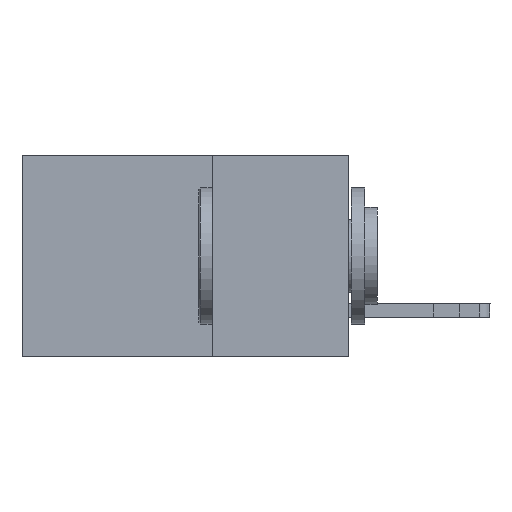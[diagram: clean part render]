
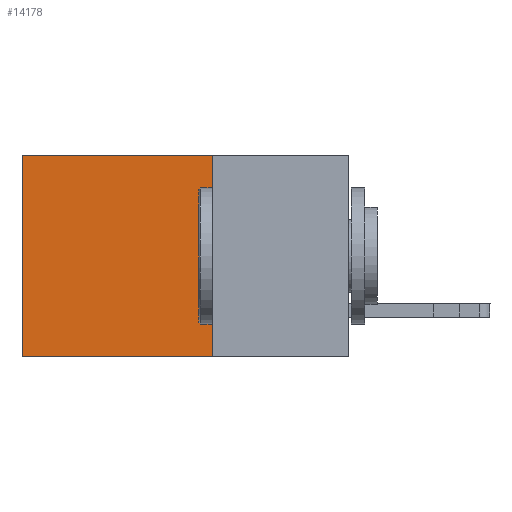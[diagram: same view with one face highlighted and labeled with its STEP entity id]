
A CAD part, left-side view. The second image highlights one B-rep face of the part: STEP entity #14178.
In plain terms, the highlighted planar face has unit normal (-1, 0, 0).
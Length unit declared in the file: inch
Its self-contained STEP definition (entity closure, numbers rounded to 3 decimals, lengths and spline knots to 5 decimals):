
#220 = VERTEX_POINT ( 'NONE', #11306 ) ;
#519 = EDGE_CURVE ( 'NONE', #220, #4418, #6284, .T. ) ;
#1216 = VECTOR ( 'NONE', #6121, 39.37008 ) ;
#1465 = CARTESIAN_POINT ( 'NONE',  ( 0.2615, 0.6, -0.37 ) ) ;
#1903 = DIRECTION ( 'NONE',  ( 1., 0., 0. ) ) ;
#2370 = VERTEX_POINT ( 'NONE', #6396 ) ;
#3082 = DIRECTION ( 'NONE',  ( 0., 1., 0. ) ) ;
#3368 = CARTESIAN_POINT ( 'NONE',  ( 0.2615, 0.25, -0.37 ) ) ;
#4298 = ORIENTED_EDGE ( 'NONE', *, *, #14673, .F. ) ;
#4418 = VERTEX_POINT ( 'NONE', #18402 ) ;
#4568 = EDGE_LOOP ( 'NONE', ( #14348, #9551, #4298, #17870 ) ) ;
#5148 = VECTOR ( 'NONE', #15956, 39.37008 ) ;
#5338 = LINE ( 'NONE', #19432, #15782 ) ;
#5769 = CARTESIAN_POINT ( 'NONE',  ( 0.2615, 0.6, -0.37 ) ) ;
#6121 = DIRECTION ( 'NONE',  ( 0., 0., -1. ) ) ;
#6284 = LINE ( 'NONE', #18919, #16658 ) ;
#6396 = CARTESIAN_POINT ( 'NONE',  ( 0.2615, 0.25, -0.37 ) ) ;
#6463 = FACE_OUTER_BOUND ( 'NONE', #4568, .T. ) ;
#9551 = ORIENTED_EDGE ( 'NONE', *, *, #16365, .F. ) ;
#9650 = CARTESIAN_POINT ( 'NONE',  ( 0.2615, 0.25, -0.37 ) ) ;
#9758 = LINE ( 'NONE', #9650, #5148 ) ;
#10227 = DIRECTION ( 'NONE',  ( 0., 1., 0. ) ) ;
#11230 = PLANE ( 'NONE',  #13404 ) ;
#11306 = CARTESIAN_POINT ( 'NONE',  ( 0.2615, 0.25, 0. ) ) ;
#13404 = AXIS2_PLACEMENT_3D ( 'NONE', #3368, #1903, #14243 ) ;
#14178 = ADVANCED_FACE ( 'NONE', ( #6463 ), #11230, .F. ) ;
#14243 = DIRECTION ( 'NONE',  ( 0., 0., -1. ) ) ;
#14348 = ORIENTED_EDGE ( 'NONE', *, *, #15687, .T. ) ;
#14673 = EDGE_CURVE ( 'NONE', #220, #2370, #9758, .T. ) ;
#15687 = EDGE_CURVE ( 'NONE', #4418, #17848, #18545, .T. ) ;
#15782 = VECTOR ( 'NONE', #10227, 39.37008 ) ;
#15956 = DIRECTION ( 'NONE',  ( 0., 0., -1. ) ) ;
#16365 = EDGE_CURVE ( 'NONE', #2370, #17848, #5338, .T. ) ;
#16658 = VECTOR ( 'NONE', #3082, 39.37008 ) ;
#17848 = VERTEX_POINT ( 'NONE', #5769 ) ;
#17870 = ORIENTED_EDGE ( 'NONE', *, *, #519, .T. ) ;
#18402 = CARTESIAN_POINT ( 'NONE',  ( 0.2615, 0.6, 0. ) ) ;
#18545 = LINE ( 'NONE', #1465, #1216 ) ;
#18919 = CARTESIAN_POINT ( 'NONE',  ( 0.2615, 0.25, 0. ) ) ;
#19432 = CARTESIAN_POINT ( 'NONE',  ( 0.2615, 0.25, -0.37 ) ) ;
